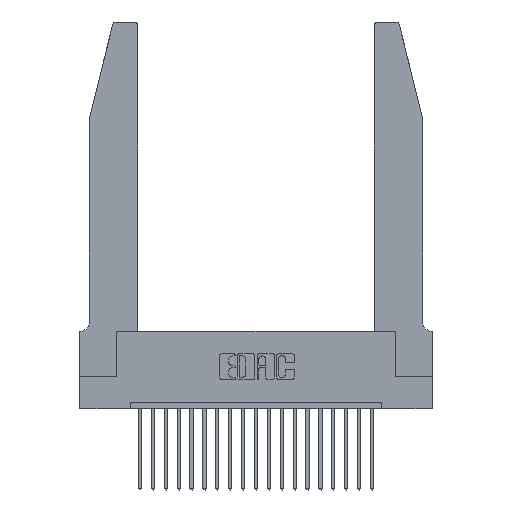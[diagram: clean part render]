
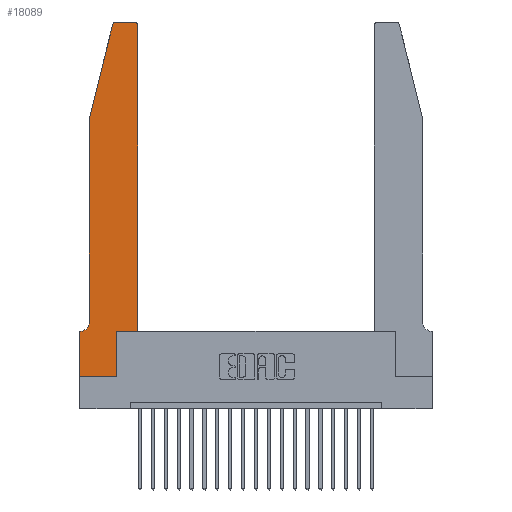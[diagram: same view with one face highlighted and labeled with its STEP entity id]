
A CAD part, top view. The second image highlights one B-rep face of the part: STEP entity #18089.
In plain terms, the highlighted planar face has unit normal (0, 0, 1).
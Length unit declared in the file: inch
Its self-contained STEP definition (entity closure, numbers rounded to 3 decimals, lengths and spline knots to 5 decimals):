
#66 = EDGE_LOOP ( 'NONE', ( #22060, #5831, #20907, #14665, #2596, #7053, #10852, #6083, #6680, #6758, #13723, #1391 ) ) ;
#374 = CARTESIAN_POINT ( 'NONE',  ( 0., 0., 0.37 ) ) ;
#406 = LINE ( 'NONE', #10064, #8348 ) ;
#1034 = VERTEX_POINT ( 'NONE', #17590 ) ;
#1391 = ORIENTED_EDGE ( 'NONE', *, *, #3708, .T. ) ;
#1415 = VECTOR ( 'NONE', #21895, 39.37008 ) ;
#1498 = LINE ( 'NONE', #10326, #1772 ) ;
#1528 = VERTEX_POINT ( 'NONE', #9362 ) ;
#1621 = CARTESIAN_POINT ( 'NONE',  ( 0.4505, 0.35, 0.37 ) ) ;
#1715 = DIRECTION ( 'NONE',  ( 1., 0., 0. ) ) ;
#1772 = VECTOR ( 'NONE', #3243, 39.37008 ) ;
#1889 = AXIS2_PLACEMENT_3D ( 'NONE', #9598, #18128, #6276 ) ;
#1948 = LINE ( 'NONE', #1621, #1415 ) ;
#2248 = CARTESIAN_POINT ( 'NONE',  ( 0.0055, 0.42, 0.37 ) ) ;
#2336 = DIRECTION ( 'NONE',  ( 0., 1., 0. ) ) ;
#2427 = CARTESIAN_POINT ( 'NONE',  ( 0.0755, 2., 0.37 ) ) ;
#2596 = ORIENTED_EDGE ( 'NONE', *, *, #6870, .T. ) ;
#2923 = EDGE_CURVE ( 'NONE', #5810, #6189, #7119, .T. ) ;
#2934 = CARTESIAN_POINT ( 'NONE',  ( 0.2605, 2.75, 0.37 ) ) ;
#3011 = FACE_OUTER_BOUND ( 'NONE', #66, .T. ) ;
#3243 = DIRECTION ( 'NONE',  ( 0., 1., 0. ) ) ;
#3297 = EDGE_CURVE ( 'NONE', #6163, #7187, #12834, .T. ) ;
#3388 = VERTEX_POINT ( 'NONE', #19277 ) ;
#3708 = EDGE_CURVE ( 'NONE', #3388, #1034, #15471, .T. ) ;
#4509 = CARTESIAN_POINT ( 'NONE',  ( 0., 0.35, 0.37 ) ) ;
#4675 = CARTESIAN_POINT ( 'NONE',  ( 0.0755, 2., 0.37 ) ) ;
#5113 = CIRCLE ( 'NONE', #18204, 0.07 ) ;
#5379 = CARTESIAN_POINT ( 'NONE',  ( 0.0055, 0.35, 0.37 ) ) ;
#5810 = VERTEX_POINT ( 'NONE', #2427 ) ;
#5831 = ORIENTED_EDGE ( 'NONE', *, *, #11542, .T. ) ;
#5925 = DIRECTION ( 'NONE',  ( 1., 0., 0. ) ) ;
#6083 = ORIENTED_EDGE ( 'NONE', *, *, #14279, .T. ) ;
#6163 = VERTEX_POINT ( 'NONE', #4509 ) ;
#6189 = VERTEX_POINT ( 'NONE', #21640 ) ;
#6276 = DIRECTION ( 'NONE',  ( 1., 0., 0. ) ) ;
#6680 = ORIENTED_EDGE ( 'NONE', *, *, #15710, .T. ) ;
#6758 = ORIENTED_EDGE ( 'NONE', *, *, #7581, .T. ) ;
#6870 = EDGE_CURVE ( 'NONE', #6189, #8677, #5113, .T. ) ;
#6991 = DIRECTION ( 'NONE',  ( 0., -1., 0. ) ) ;
#7053 = ORIENTED_EDGE ( 'NONE', *, *, #16678, .T. ) ;
#7119 = LINE ( 'NONE', #4675, #7671 ) ;
#7187 = VERTEX_POINT ( 'NONE', #10693 ) ;
#7581 = EDGE_CURVE ( 'NONE', #18418, #14914, #1948, .T. ) ;
#7671 = VECTOR ( 'NONE', #11835, 39.37008 ) ;
#7746 = CARTESIAN_POINT ( 'NONE',  ( 0.284, 2.72, 0.37 ) ) ;
#7887 = DIRECTION ( 'NONE',  ( 0., 0., 1. ) ) ;
#8348 = VECTOR ( 'NONE', #16876, 39.37008 ) ;
#8360 = VECTOR ( 'NONE', #18181, 39.37008 ) ;
#8609 = CARTESIAN_POINT ( 'NONE',  ( 0.4505, 0.35, 0.37 ) ) ;
#8650 = CARTESIAN_POINT ( 'NONE',  ( 0.2865, 0.35, 0.37 ) ) ;
#8677 = VERTEX_POINT ( 'NONE', #5379 ) ;
#9034 = DIRECTION ( 'NONE',  ( -1., 0., 0. ) ) ;
#9165 = EDGE_CURVE ( 'NONE', #1034, #21581, #12206, .T. ) ;
#9362 = CARTESIAN_POINT ( 'NONE',  ( 0.25487, 2.72718, 0.37 ) ) ;
#9598 = CARTESIAN_POINT ( 'NONE',  ( 0., 0.35, 0.37 ) ) ;
#9628 = LINE ( 'NONE', #19385, #13117 ) ;
#10064 = CARTESIAN_POINT ( 'NONE',  ( 0.0755, 2., 0.37 ) ) ;
#10326 = CARTESIAN_POINT ( 'NONE',  ( 0.2865, 0.35, 0.37 ) ) ;
#10693 = CARTESIAN_POINT ( 'NONE',  ( 0., 0., 0.37 ) ) ;
#10852 = ORIENTED_EDGE ( 'NONE', *, *, #3297, .T. ) ;
#11353 = EDGE_CURVE ( 'NONE', #14914, #3388, #9628, .T. ) ;
#11542 = EDGE_CURVE ( 'NONE', #21581, #1528, #12880, .T. ) ;
#11718 = CARTESIAN_POINT ( 'NONE',  ( 0.4205, 2.72, 0.37 ) ) ;
#11835 = DIRECTION ( 'NONE',  ( 0., -1., 0. ) ) ;
#12206 = LINE ( 'NONE', #2934, #8360 ) ;
#12834 = LINE ( 'NONE', #374, #17650 ) ;
#12880 = CIRCLE ( 'NONE', #13827, 0.03 ) ;
#13117 = VECTOR ( 'NONE', #2336, 39.37008 ) ;
#13284 = LINE ( 'NONE', #13931, #13839 ) ;
#13723 = ORIENTED_EDGE ( 'NONE', *, *, #11353, .T. ) ;
#13827 = AXIS2_PLACEMENT_3D ( 'NONE', #7746, #14422, #5925 ) ;
#13839 = VECTOR ( 'NONE', #1715, 39.37008 ) ;
#13931 = CARTESIAN_POINT ( 'NONE',  ( 0., 0., 0.37 ) ) ;
#14175 = AXIS2_PLACEMENT_3D ( 'NONE', #11718, #7887, #17891 ) ;
#14207 = CARTESIAN_POINT ( 'NONE',  ( 0.284, 2.75, 0.37 ) ) ;
#14279 = EDGE_CURVE ( 'NONE', #7187, #16886, #13284, .T. ) ;
#14422 = DIRECTION ( 'NONE',  ( 0., 0., 1. ) ) ;
#14665 = ORIENTED_EDGE ( 'NONE', *, *, #2923, .T. ) ;
#14914 = VERTEX_POINT ( 'NONE', #8609 ) ;
#15471 = CIRCLE ( 'NONE', #14175, 0.03 ) ;
#15710 = EDGE_CURVE ( 'NONE', #16886, #18418, #1498, .T. ) ;
#15934 = DIRECTION ( 'NONE',  ( 0., 0., -1. ) ) ;
#16667 = CARTESIAN_POINT ( 'NONE',  ( 0.2865, 0., 0.37 ) ) ;
#16678 = EDGE_CURVE ( 'NONE', #8677, #6163, #18568, .T. ) ;
#16876 = DIRECTION ( 'NONE',  ( -0.239, -0.971, 0. ) ) ;
#16886 = VERTEX_POINT ( 'NONE', #16667 ) ;
#17524 = EDGE_CURVE ( 'NONE', #1528, #5810, #406, .T. ) ;
#17590 = CARTESIAN_POINT ( 'NONE',  ( 0.4205, 2.75, 0.37 ) ) ;
#17650 = VECTOR ( 'NONE', #6991, 39.37008 ) ;
#17891 = DIRECTION ( 'NONE',  ( 1., 0., 0. ) ) ;
#18038 = CARTESIAN_POINT ( 'NONE',  ( 0.0755, 0.35, 0.37 ) ) ;
#18089 = ADVANCED_FACE ( 'NONE', ( #3011 ), #21650, .T. ) ;
#18128 = DIRECTION ( 'NONE',  ( 0., 0., 1. ) ) ;
#18181 = DIRECTION ( 'NONE',  ( -1., 0., 0. ) ) ;
#18204 = AXIS2_PLACEMENT_3D ( 'NONE', #2248, #15934, #9034 ) ;
#18418 = VERTEX_POINT ( 'NONE', #8650 ) ;
#18568 = LINE ( 'NONE', #18038, #21274 ) ;
#19277 = CARTESIAN_POINT ( 'NONE',  ( 0.4505, 2.72, 0.37 ) ) ;
#19385 = CARTESIAN_POINT ( 'NONE',  ( 0.4505, 0.35, 0.37 ) ) ;
#20907 = ORIENTED_EDGE ( 'NONE', *, *, #17524, .T. ) ;
#20949 = DIRECTION ( 'NONE',  ( -1., 0., 0. ) ) ;
#21274 = VECTOR ( 'NONE', #20949, 39.37008 ) ;
#21581 = VERTEX_POINT ( 'NONE', #14207 ) ;
#21640 = CARTESIAN_POINT ( 'NONE',  ( 0.0755, 0.42, 0.37 ) ) ;
#21650 = PLANE ( 'NONE',  #1889 ) ;
#21895 = DIRECTION ( 'NONE',  ( 1., 0., 0. ) ) ;
#22060 = ORIENTED_EDGE ( 'NONE', *, *, #9165, .T. ) ;
